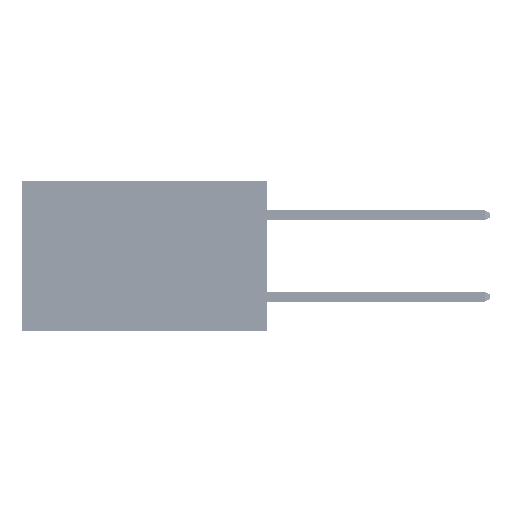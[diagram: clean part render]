
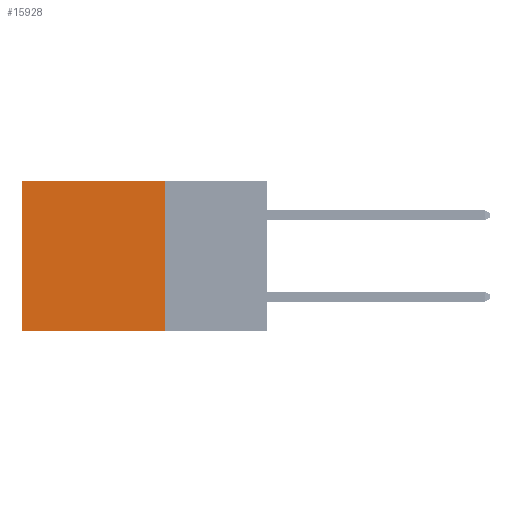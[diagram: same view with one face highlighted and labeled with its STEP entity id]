
A CAD part, left-side view. The second image highlights one B-rep face of the part: STEP entity #15928.
In plain terms, the highlighted planar face has unit normal (-1, 0, 0).
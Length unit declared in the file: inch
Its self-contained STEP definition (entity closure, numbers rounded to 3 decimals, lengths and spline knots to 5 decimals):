
#2545 = ORIENTED_EDGE ( 'NONE', *, *, #33457, .T. ) ;
#3709 = EDGE_CURVE ( 'NONE', #35065, #30888, #3903, .T. ) ;
#3903 = LINE ( 'NONE', #38733, #33794 ) ;
#6826 = VECTOR ( 'NONE', #19672, 39.37008 ) ;
#10631 = CARTESIAN_POINT ( 'NONE',  ( 0.2875, 0.6, -0.37 ) ) ;
#11739 = AXIS2_PLACEMENT_3D ( 'NONE', #37582, #23016, #18771 ) ;
#12248 = CARTESIAN_POINT ( 'NONE',  ( 0.2875, 0.25, 0. ) ) ;
#15928 = ADVANCED_FACE ( 'NONE', ( #22064 ), #36814, .F. ) ;
#16282 = EDGE_CURVE ( 'NONE', #44891, #25362, #17341, .T. ) ;
#16718 = VECTOR ( 'NONE', #39994, 39.37008 ) ;
#17341 = LINE ( 'NONE', #28200, #16718 ) ;
#18771 = DIRECTION ( 'NONE',  ( 0., 0., -1. ) ) ;
#19654 = ORIENTED_EDGE ( 'NONE', *, *, #3709, .F. ) ;
#19672 = DIRECTION ( 'NONE',  ( 0., 0., -1. ) ) ;
#19865 = CARTESIAN_POINT ( 'NONE',  ( 0.2875, 0.25, -0.37 ) ) ;
#22064 = FACE_OUTER_BOUND ( 'NONE', #33612, .T. ) ;
#23016 = DIRECTION ( 'NONE',  ( 1., 0., 0. ) ) ;
#24552 = CARTESIAN_POINT ( 'NONE',  ( 0.2875, 0.6, 0. ) ) ;
#25362 = VERTEX_POINT ( 'NONE', #32825 ) ;
#27326 = VECTOR ( 'NONE', #32053, 39.37008 ) ;
#28200 = CARTESIAN_POINT ( 'NONE',  ( 0.2875, 0.25, 0. ) ) ;
#28957 = ORIENTED_EDGE ( 'NONE', *, *, #33290, .F. ) ;
#30888 = VERTEX_POINT ( 'NONE', #10631 ) ;
#31989 = LINE ( 'NONE', #24552, #27326 ) ;
#32053 = DIRECTION ( 'NONE',  ( 0., 0., -1. ) ) ;
#32825 = CARTESIAN_POINT ( 'NONE',  ( 0.2875, 0.6, 0. ) ) ;
#33290 = EDGE_CURVE ( 'NONE', #44891, #35065, #37335, .T. ) ;
#33457 = EDGE_CURVE ( 'NONE', #25362, #30888, #31989, .T. ) ;
#33612 = EDGE_LOOP ( 'NONE', ( #2545, #19654, #28957, #36858 ) ) ;
#33794 = VECTOR ( 'NONE', #38888, 39.37008 ) ;
#35065 = VERTEX_POINT ( 'NONE', #19865 ) ;
#36424 = CARTESIAN_POINT ( 'NONE',  ( 0.2875, 0.25, 0. ) ) ;
#36814 = PLANE ( 'NONE',  #11739 ) ;
#36858 = ORIENTED_EDGE ( 'NONE', *, *, #16282, .T. ) ;
#37335 = LINE ( 'NONE', #12248, #6826 ) ;
#37582 = CARTESIAN_POINT ( 'NONE',  ( 0.2875, 0.25, 0. ) ) ;
#38733 = CARTESIAN_POINT ( 'NONE',  ( 0.2875, 0.25, -0.37 ) ) ;
#38888 = DIRECTION ( 'NONE',  ( 0., 1., 0. ) ) ;
#39994 = DIRECTION ( 'NONE',  ( 0., 1., 0. ) ) ;
#44891 = VERTEX_POINT ( 'NONE', #36424 ) ;
